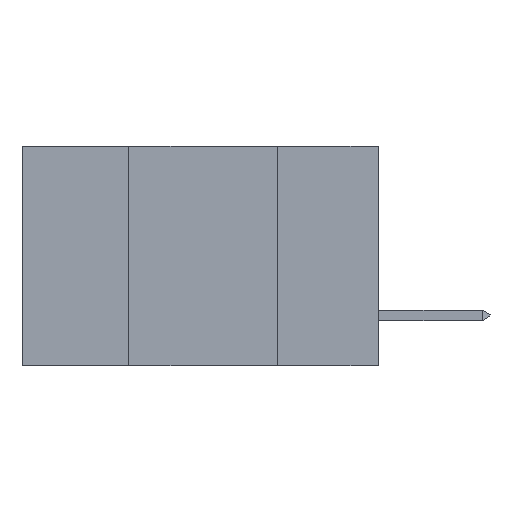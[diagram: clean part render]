
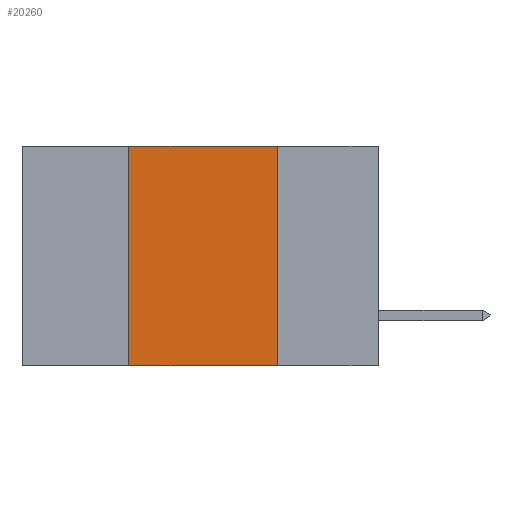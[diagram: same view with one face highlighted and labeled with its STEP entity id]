
A CAD part, left-side view. The second image highlights one B-rep face of the part: STEP entity #20260.
In plain terms, the highlighted planar face has unit normal (-1, 0, 0).
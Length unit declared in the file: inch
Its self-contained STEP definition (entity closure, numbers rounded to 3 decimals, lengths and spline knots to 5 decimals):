
#64 = EDGE_LOOP ( 'NONE', ( #8999, #5709, #11220, #6331 ) ) ;
#1234 = EDGE_CURVE ( 'NONE', #10314, #21816, #4646, .T. ) ;
#2203 = LINE ( 'NONE', #11153, #11869 ) ;
#2240 = DIRECTION ( 'NONE',  ( 0., 0., -1. ) ) ;
#3200 = LINE ( 'NONE', #10381, #16841 ) ;
#4026 = EDGE_CURVE ( 'NONE', #15773, #21816, #2203, .T. ) ;
#4646 = LINE ( 'NONE', #11830, #15210 ) ;
#5163 = LINE ( 'NONE', #10588, #17976 ) ;
#5509 = DIRECTION ( 'NONE',  ( 0., 0., 1. ) ) ;
#5694 = VERTEX_POINT ( 'NONE', #16422 ) ;
#5709 = ORIENTED_EDGE ( 'NONE', *, *, #16404, .F. ) ;
#6331 = ORIENTED_EDGE ( 'NONE', *, *, #1234, .T. ) ;
#6529 = DIRECTION ( 'NONE',  ( 0., -1., 0. ) ) ;
#6744 = AXIS2_PLACEMENT_3D ( 'NONE', #22002, #13060, #2240 ) ;
#7622 = DIRECTION ( 'NONE',  ( 0., 0., -1. ) ) ;
#8999 = ORIENTED_EDGE ( 'NONE', *, *, #4026, .F. ) ;
#9192 = PLANE ( 'NONE',  #6744 ) ;
#9708 = CARTESIAN_POINT ( 'NONE',  ( 0., 0.17, 0. ) ) ;
#10314 = VERTEX_POINT ( 'NONE', #14636 ) ;
#10381 = CARTESIAN_POINT ( 'NONE',  ( 0., 0.6, 0. ) ) ;
#10588 = CARTESIAN_POINT ( 'NONE',  ( 0., 0.42, -0.37 ) ) ;
#11153 = CARTESIAN_POINT ( 'NONE',  ( 0., 0.17, -0.37 ) ) ;
#11220 = ORIENTED_EDGE ( 'NONE', *, *, #16964, .F. ) ;
#11830 = CARTESIAN_POINT ( 'NONE',  ( 0., 0.6, -0.37 ) ) ;
#11869 = VECTOR ( 'NONE', #7622, 39.37008 ) ;
#13060 = DIRECTION ( 'NONE',  ( 1., 0., 0. ) ) ;
#14022 = DIRECTION ( 'NONE',  ( 0., -1., 0. ) ) ;
#14636 = CARTESIAN_POINT ( 'NONE',  ( 0., 0.42, -0.37 ) ) ;
#15210 = VECTOR ( 'NONE', #6529, 39.37008 ) ;
#15773 = VERTEX_POINT ( 'NONE', #9708 ) ;
#16404 = EDGE_CURVE ( 'NONE', #5694, #15773, #3200, .T. ) ;
#16422 = CARTESIAN_POINT ( 'NONE',  ( 0., 0.42, 0. ) ) ;
#16841 = VECTOR ( 'NONE', #14022, 39.37008 ) ;
#16964 = EDGE_CURVE ( 'NONE', #10314, #5694, #5163, .T. ) ;
#17634 = CARTESIAN_POINT ( 'NONE',  ( 0., 0.17, -0.37 ) ) ;
#17976 = VECTOR ( 'NONE', #5509, 39.37008 ) ;
#18233 = FACE_OUTER_BOUND ( 'NONE', #64, .T. ) ;
#20260 = ADVANCED_FACE ( 'NONE', ( #18233 ), #9192, .F. ) ;
#21816 = VERTEX_POINT ( 'NONE', #17634 ) ;
#22002 = CARTESIAN_POINT ( 'NONE',  ( 0., 0.6, 0. ) ) ;
